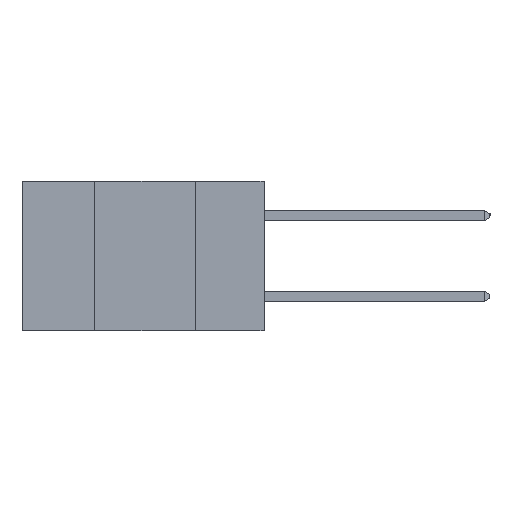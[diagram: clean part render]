
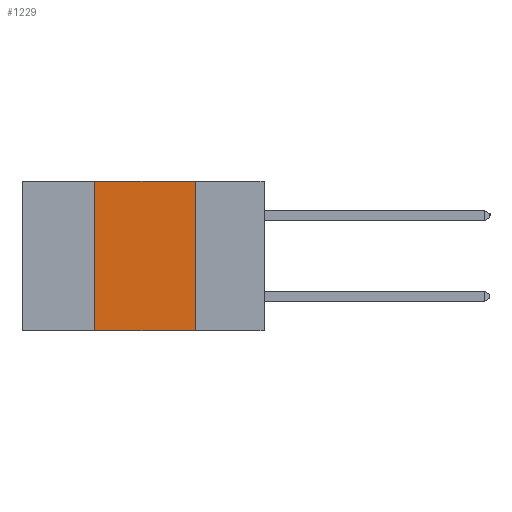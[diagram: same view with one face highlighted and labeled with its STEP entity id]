
A CAD part, left-side view. The second image highlights one B-rep face of the part: STEP entity #1229.
In plain terms, the highlighted planar face has unit normal (-1, 0, 0).
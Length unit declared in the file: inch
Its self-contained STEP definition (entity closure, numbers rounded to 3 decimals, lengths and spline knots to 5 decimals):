
#71 = CARTESIAN_POINT ( 'NONE',  ( 0., 0.17, -0.37 ) ) ;
#405 = CARTESIAN_POINT ( 'NONE',  ( 0., 0.17, 0. ) ) ;
#1229 = ADVANCED_FACE ( 'NONE', ( #12550 ), #2094, .F. ) ;
#1867 = ORIENTED_EDGE ( 'NONE', *, *, #3885, .T. ) ;
#2094 = PLANE ( 'NONE',  #13713 ) ;
#2318 = ORIENTED_EDGE ( 'NONE', *, *, #17149, .F. ) ;
#2342 = VERTEX_POINT ( 'NONE', #5313 ) ;
#2615 = VERTEX_POINT ( 'NONE', #14205 ) ;
#2907 = VERTEX_POINT ( 'NONE', #4578 ) ;
#3885 = EDGE_CURVE ( 'NONE', #2342, #2615, #16453, .T. ) ;
#4578 = CARTESIAN_POINT ( 'NONE',  ( 0., 0.42, 0. ) ) ;
#4842 = CARTESIAN_POINT ( 'NONE',  ( 0., 0.6, -0.37 ) ) ;
#5313 = CARTESIAN_POINT ( 'NONE',  ( 0., 0.42, -0.37 ) ) ;
#5707 = VECTOR ( 'NONE', #17371, 39.37008 ) ;
#6146 = VECTOR ( 'NONE', #11217, 39.37008 ) ;
#6226 = DIRECTION ( 'NONE',  ( 0., 0., -1. ) ) ;
#6809 = VERTEX_POINT ( 'NONE', #405 ) ;
#8034 = LINE ( 'NONE', #9668, #6146 ) ;
#8227 = CARTESIAN_POINT ( 'NONE',  ( 0., 0.6, 0. ) ) ;
#8241 = EDGE_LOOP ( 'NONE', ( #16173, #16903, #2318, #1867 ) ) ;
#9345 = VECTOR ( 'NONE', #6226, 39.37008 ) ;
#9668 = CARTESIAN_POINT ( 'NONE',  ( 0., 0.42, -0.37 ) ) ;
#10693 = DIRECTION ( 'NONE',  ( 0., -1., 0. ) ) ;
#11217 = DIRECTION ( 'NONE',  ( 0., 0., 1. ) ) ;
#11236 = LINE ( 'NONE', #14317, #5707 ) ;
#11800 = LINE ( 'NONE', #71, #9345 ) ;
#12364 = EDGE_CURVE ( 'NONE', #6809, #2615, #11800, .T. ) ;
#12550 = FACE_OUTER_BOUND ( 'NONE', #8241, .T. ) ;
#13713 = AXIS2_PLACEMENT_3D ( 'NONE', #8227, #18236, #14011 ) ;
#14011 = DIRECTION ( 'NONE',  ( 0., 0., -1. ) ) ;
#14205 = CARTESIAN_POINT ( 'NONE',  ( 0., 0.17, -0.37 ) ) ;
#14317 = CARTESIAN_POINT ( 'NONE',  ( 0., 0.6, 0. ) ) ;
#15286 = EDGE_CURVE ( 'NONE', #2907, #6809, #11236, .T. ) ;
#16173 = ORIENTED_EDGE ( 'NONE', *, *, #12364, .F. ) ;
#16453 = LINE ( 'NONE', #4842, #17511 ) ;
#16903 = ORIENTED_EDGE ( 'NONE', *, *, #15286, .F. ) ;
#17149 = EDGE_CURVE ( 'NONE', #2342, #2907, #8034, .T. ) ;
#17371 = DIRECTION ( 'NONE',  ( 0., -1., 0. ) ) ;
#17511 = VECTOR ( 'NONE', #10693, 39.37008 ) ;
#18236 = DIRECTION ( 'NONE',  ( 1., 0., 0. ) ) ;
